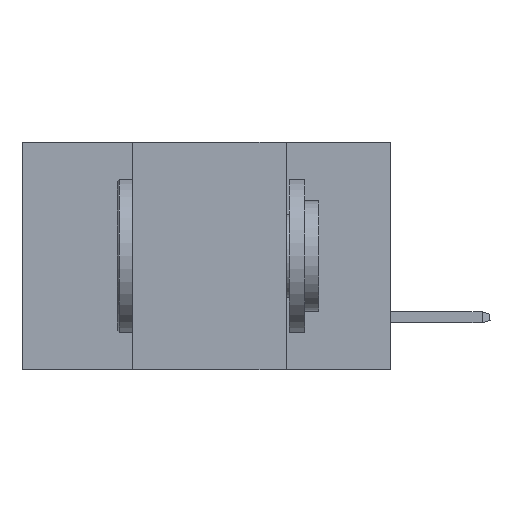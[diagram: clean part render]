
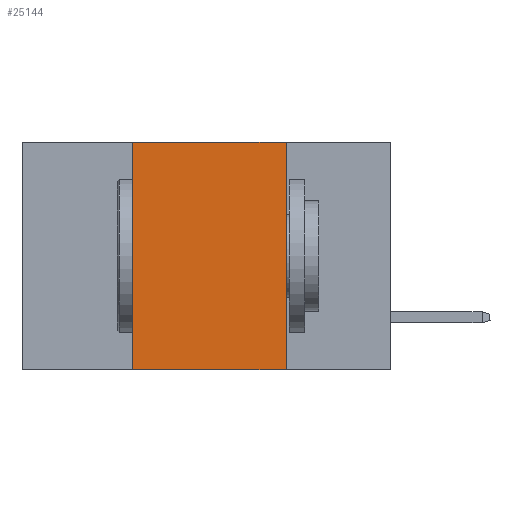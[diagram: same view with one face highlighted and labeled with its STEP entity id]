
A CAD part, left-side view. The second image highlights one B-rep face of the part: STEP entity #25144.
In plain terms, the highlighted planar face has unit normal (-1, 0, 0).
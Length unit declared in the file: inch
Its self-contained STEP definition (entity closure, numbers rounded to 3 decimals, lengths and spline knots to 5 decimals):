
#702 = LINE ( 'NONE', #10198, #13820 ) ;
#1749 = EDGE_CURVE ( 'NONE', #10732, #15692, #10399, .T. ) ;
#1904 = EDGE_CURVE ( 'NONE', #7023, #10732, #6898, .T. ) ;
#4322 = CARTESIAN_POINT ( 'NONE',  ( 0., 0.42, 0. ) ) ;
#5038 = EDGE_CURVE ( 'NONE', #15692, #8180, #702, .T. ) ;
#5626 = CARTESIAN_POINT ( 'NONE',  ( 0., 0.6, 0. ) ) ;
#6128 = EDGE_LOOP ( 'NONE', ( #16903, #20984, #28527, #17250 ) ) ;
#6898 = LINE ( 'NONE', #4322, #12446 ) ;
#7023 = VERTEX_POINT ( 'NONE', #21374 ) ;
#8180 = VERTEX_POINT ( 'NONE', #12197 ) ;
#10198 = CARTESIAN_POINT ( 'NONE',  ( 0., 0.17, 0. ) ) ;
#10399 = LINE ( 'NONE', #5626, #12478 ) ;
#10732 = VERTEX_POINT ( 'NONE', #12219 ) ;
#12135 = CARTESIAN_POINT ( 'NONE',  ( 0., 0.6, -0.37 ) ) ;
#12197 = CARTESIAN_POINT ( 'NONE',  ( 0., 0.17, -0.37 ) ) ;
#12219 = CARTESIAN_POINT ( 'NONE',  ( 0., 0.42, 0. ) ) ;
#12446 = VECTOR ( 'NONE', #25325, 39.37008 ) ;
#12478 = VECTOR ( 'NONE', #16510, 39.37008 ) ;
#13178 = DIRECTION ( 'NONE',  ( 1., 0., 0. ) ) ;
#13275 = DIRECTION ( 'NONE',  ( 0., 0., -1. ) ) ;
#13820 = VECTOR ( 'NONE', #14710, 39.37008 ) ;
#14135 = FACE_OUTER_BOUND ( 'NONE', #6128, .T. ) ;
#14710 = DIRECTION ( 'NONE',  ( 0., 0., -1. ) ) ;
#15692 = VERTEX_POINT ( 'NONE', #16061 ) ;
#16061 = CARTESIAN_POINT ( 'NONE',  ( 0., 0.17, 0. ) ) ;
#16510 = DIRECTION ( 'NONE',  ( 0., -1., 0. ) ) ;
#16903 = ORIENTED_EDGE ( 'NONE', *, *, #5038, .F. ) ;
#17015 = LINE ( 'NONE', #12135, #27131 ) ;
#17159 = PLANE ( 'NONE',  #22528 ) ;
#17250 = ORIENTED_EDGE ( 'NONE', *, *, #27852, .T. ) ;
#20984 = ORIENTED_EDGE ( 'NONE', *, *, #1749, .F. ) ;
#21374 = CARTESIAN_POINT ( 'NONE',  ( 0., 0.42, -0.37 ) ) ;
#22528 = AXIS2_PLACEMENT_3D ( 'NONE', #28768, #13178, #13275 ) ;
#25144 = ADVANCED_FACE ( 'NONE', ( #14135 ), #17159, .F. ) ;
#25325 = DIRECTION ( 'NONE',  ( 0., 0., 1. ) ) ;
#25373 = DIRECTION ( 'NONE',  ( 0., -1., 0. ) ) ;
#27131 = VECTOR ( 'NONE', #25373, 39.37008 ) ;
#27852 = EDGE_CURVE ( 'NONE', #7023, #8180, #17015, .T. ) ;
#28527 = ORIENTED_EDGE ( 'NONE', *, *, #1904, .F. ) ;
#28768 = CARTESIAN_POINT ( 'NONE',  ( 0., 0.6, 0. ) ) ;
